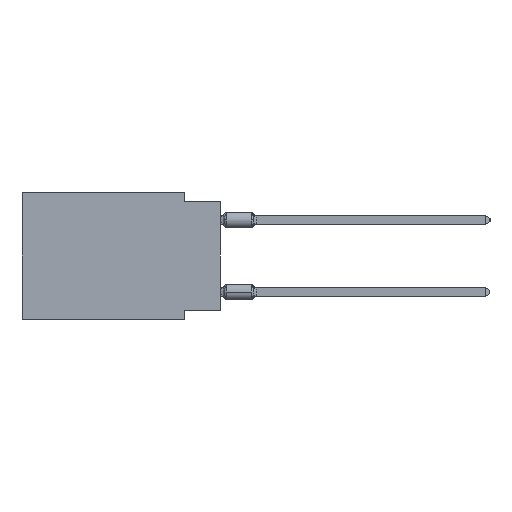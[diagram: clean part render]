
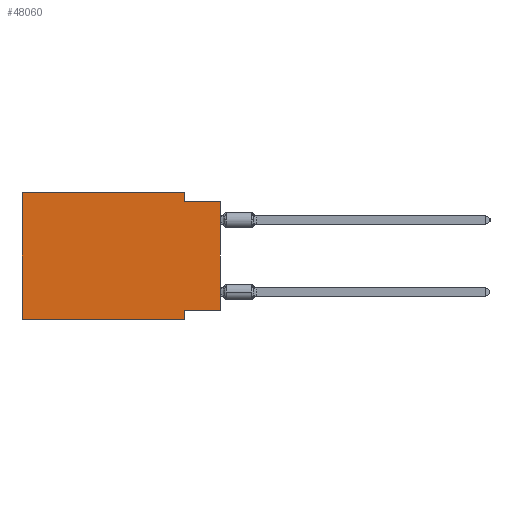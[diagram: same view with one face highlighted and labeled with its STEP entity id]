
A CAD part, left-side view. The second image highlights one B-rep face of the part: STEP entity #48060.
In plain terms, the highlighted planar face has unit normal (-1, 0, 0).
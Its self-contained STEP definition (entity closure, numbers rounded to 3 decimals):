
#1912 = ORIENTED_EDGE ( 'NONE', *, *, #30304, .T. ) ;
#4563 = VERTEX_POINT ( 'NONE', #47945 ) ;
#5141 = DIRECTION ( 'NONE',  ( 0., 0., 1. ) ) ;
#5667 = CARTESIAN_POINT ( 'NONE',  ( 0., 13.97, -8.89 ) ) ;
#5905 = VECTOR ( 'NONE', #5141, 1000. ) ;
#6369 = VECTOR ( 'NONE', #36175, 1000. ) ;
#7324 = ORIENTED_EDGE ( 'NONE', *, *, #25060, .F. ) ;
#8608 = DIRECTION ( 'NONE',  ( 1., 0., 0. ) ) ;
#9785 = ORIENTED_EDGE ( 'NONE', *, *, #25855, .F. ) ;
#10159 = EDGE_CURVE ( 'NONE', #4563, #22973, #21482, .T. ) ;
#11262 = DIRECTION ( 'NONE',  ( 0., 0., -1. ) ) ;
#12493 = CARTESIAN_POINT ( 'NONE',  ( 0., 13.97, 0. ) ) ;
#13780 = DIRECTION ( 'NONE',  ( 0., 1., 0. ) ) ;
#13965 = DIRECTION ( 'NONE',  ( 0., 0., 1. ) ) ;
#14650 = LINE ( 'NONE', #45456, #24438 ) ;
#18050 = ORIENTED_EDGE ( 'NONE', *, *, #10159, .F. ) ;
#18530 = CARTESIAN_POINT ( 'NONE',  ( 0., 13.97, 0. ) ) ;
#18884 = CARTESIAN_POINT ( 'NONE',  ( 0., 2.54, -8.255 ) ) ;
#18981 = VERTEX_POINT ( 'NONE', #21261 ) ;
#20962 = VECTOR ( 'NONE', #38915, 1000. ) ;
#21238 = CARTESIAN_POINT ( 'NONE',  ( 0., 0., -0.635 ) ) ;
#21261 = CARTESIAN_POINT ( 'NONE',  ( 0., 13.97, 0. ) ) ;
#21482 = LINE ( 'NONE', #43274, #6369 ) ;
#21860 = CARTESIAN_POINT ( 'NONE',  ( 0., 2.54, 0. ) ) ;
#22973 = VERTEX_POINT ( 'NONE', #21238 ) ;
#24141 = ORIENTED_EDGE ( 'NONE', *, *, #31727, .F. ) ;
#24438 = VECTOR ( 'NONE', #11262, 1000. ) ;
#25019 = CARTESIAN_POINT ( 'NONE',  ( 0., 0., -8.255 ) ) ;
#25060 = EDGE_CURVE ( 'NONE', #35951, #18981, #31069, .T. ) ;
#25855 = EDGE_CURVE ( 'NONE', #36042, #28447, #26137, .T. ) ;
#25880 = EDGE_CURVE ( 'NONE', #18981, #47505, #30286, .T. ) ;
#26025 = ORIENTED_EDGE ( 'NONE', *, *, #28535, .T. ) ;
#26137 = LINE ( 'NONE', #26374, #43463 ) ;
#26374 = CARTESIAN_POINT ( 'NONE',  ( 0., 2.54, -8.89 ) ) ;
#26644 = EDGE_LOOP ( 'NONE', ( #1912, #18050, #38160, #45207, #7324, #26025, #9785, #24141 ) ) ;
#27043 = VECTOR ( 'NONE', #13965, 1000. ) ;
#27430 = CARTESIAN_POINT ( 'NONE',  ( 0., 13.97, 0. ) ) ;
#27921 = CARTESIAN_POINT ( 'NONE',  ( 0., 2.54, -8.89 ) ) ;
#28447 = VERTEX_POINT ( 'NONE', #27921 ) ;
#28535 = EDGE_CURVE ( 'NONE', #35951, #28447, #39158, .T. ) ;
#29122 = CARTESIAN_POINT ( 'NONE',  ( 0., 0., 0. ) ) ;
#30286 = LINE ( 'NONE', #18530, #45808 ) ;
#30304 = EDGE_CURVE ( 'NONE', #45696, #22973, #32540, .T. ) ;
#30385 = PLANE ( 'NONE',  #40633 ) ;
#31069 = LINE ( 'NONE', #12493, #5905 ) ;
#31337 = DIRECTION ( 'NONE',  ( 0., 0., -1. ) ) ;
#31727 = EDGE_CURVE ( 'NONE', #45696, #36042, #33078, .T. ) ;
#32540 = LINE ( 'NONE', #29122, #27043 ) ;
#33078 = LINE ( 'NONE', #25019, #42150 ) ;
#33449 = DIRECTION ( 'NONE',  ( 0., -1., 0. ) ) ;
#34927 = CARTESIAN_POINT ( 'NONE',  ( 0., 0., -8.255 ) ) ;
#35951 = VERTEX_POINT ( 'NONE', #44078 ) ;
#36042 = VERTEX_POINT ( 'NONE', #18884 ) ;
#36175 = DIRECTION ( 'NONE',  ( 0., -1., 0. ) ) ;
#36733 = DIRECTION ( 'NONE',  ( 0., 0., -1. ) ) ;
#38160 = ORIENTED_EDGE ( 'NONE', *, *, #45544, .F. ) ;
#38915 = DIRECTION ( 'NONE',  ( 0., -1., 0. ) ) ;
#39158 = LINE ( 'NONE', #5667, #20962 ) ;
#40633 = AXIS2_PLACEMENT_3D ( 'NONE', #27430, #8608, #31337 ) ;
#42150 = VECTOR ( 'NONE', #13780, 1000. ) ;
#43274 = CARTESIAN_POINT ( 'NONE',  ( 0., 0., -0.635 ) ) ;
#43463 = VECTOR ( 'NONE', #36733, 1000. ) ;
#44078 = CARTESIAN_POINT ( 'NONE',  ( 0., 13.97, -8.89 ) ) ;
#45207 = ORIENTED_EDGE ( 'NONE', *, *, #25880, .F. ) ;
#45456 = CARTESIAN_POINT ( 'NONE',  ( 0., 2.54, 0. ) ) ;
#45544 = EDGE_CURVE ( 'NONE', #47505, #4563, #14650, .T. ) ;
#45696 = VERTEX_POINT ( 'NONE', #34927 ) ;
#45764 = FACE_OUTER_BOUND ( 'NONE', #26644, .T. ) ;
#45808 = VECTOR ( 'NONE', #33449, 1000. ) ;
#47505 = VERTEX_POINT ( 'NONE', #21860 ) ;
#47945 = CARTESIAN_POINT ( 'NONE',  ( 0., 2.54, -0.635 ) ) ;
#48060 = ADVANCED_FACE ( 'NONE', ( #45764 ), #30385, .F. ) ;
